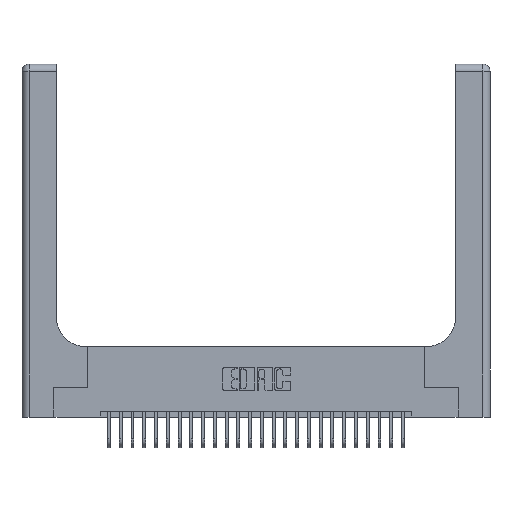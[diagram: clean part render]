
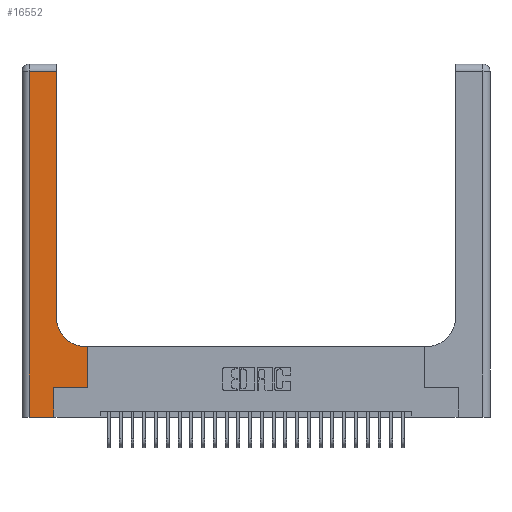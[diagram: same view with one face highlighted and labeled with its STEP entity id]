
A CAD part, top view. The second image highlights one B-rep face of the part: STEP entity #16552.
In plain terms, the highlighted planar face has unit normal (0, 0, 1).
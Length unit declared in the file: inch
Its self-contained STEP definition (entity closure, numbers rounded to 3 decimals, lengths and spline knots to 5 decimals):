
#147 = CARTESIAN_POINT ( 'NONE',  ( 0.269, 0.25, 0.37 ) ) ;
#565 = DIRECTION ( 'NONE',  ( 0., 1., 0. ) ) ;
#669 = ORIENTED_EDGE ( 'NONE', *, *, #23803, .T. ) ;
#1334 = ORIENTED_EDGE ( 'NONE', *, *, #16350, .T. ) ;
#1658 = CARTESIAN_POINT ( 'NONE',  ( 0.2915, 3., 0.37 ) ) ;
#2383 = PLANE ( 'NONE',  #17959 ) ;
#2722 = LINE ( 'NONE', #16464, #17985 ) ;
#2765 = CARTESIAN_POINT ( 'NONE',  ( 0.269, 0., 0.37 ) ) ;
#3053 = EDGE_CURVE ( 'NONE', #5883, #18061, #13501, .T. ) ;
#3487 = CARTESIAN_POINT ( 'NONE',  ( 0.2915, 0.6, 0.37 ) ) ;
#3975 = CARTESIAN_POINT ( 'NONE',  ( 0.2915, 0.85, 0.37 ) ) ;
#4503 = DIRECTION ( 'NONE',  ( -1., 0., 0. ) ) ;
#4833 = LINE ( 'NONE', #11302, #15850 ) ;
#5059 = VERTEX_POINT ( 'NONE', #21029 ) ;
#5406 = FACE_OUTER_BOUND ( 'NONE', #20144, .T. ) ;
#5521 = CARTESIAN_POINT ( 'NONE',  ( 0.5415, 0.6, 0.37 ) ) ;
#5648 = CIRCLE ( 'NONE', #12355, 0.25 ) ;
#5775 = LINE ( 'NONE', #18888, #20976 ) ;
#5845 = VERTEX_POINT ( 'NONE', #2765 ) ;
#5883 = VERTEX_POINT ( 'NONE', #11159 ) ;
#6064 = EDGE_CURVE ( 'NONE', #14129, #5845, #2722, .T. ) ;
#6134 = DIRECTION ( 'NONE',  ( 1., 0., 0. ) ) ;
#7272 = ORIENTED_EDGE ( 'NONE', *, *, #6064, .T. ) ;
#7754 = CARTESIAN_POINT ( 'NONE',  ( 0.5415, 0.85, 0.37 ) ) ;
#7969 = DIRECTION ( 'NONE',  ( 0., 1., 0. ) ) ;
#8744 = VECTOR ( 'NONE', #7969, 39.37008 ) ;
#9002 = EDGE_CURVE ( 'NONE', #21495, #17935, #11755, .T. ) ;
#9151 = CARTESIAN_POINT ( 'NONE',  ( 0.269, 0.25, 0.37 ) ) ;
#9837 = DIRECTION ( 'NONE',  ( 1., 0., 0. ) ) ;
#11151 = ORIENTED_EDGE ( 'NONE', *, *, #9002, .T. ) ;
#11159 = CARTESIAN_POINT ( 'NONE',  ( 0.5585, 0.6, 0.37 ) ) ;
#11218 = DIRECTION ( 'NONE',  ( 1., 0., 0. ) ) ;
#11302 = CARTESIAN_POINT ( 'NONE',  ( 0.06, 3., 0.37 ) ) ;
#11467 = VECTOR ( 'NONE', #565, 39.37008 ) ;
#11755 = LINE ( 'NONE', #9151, #15922 ) ;
#12114 = LINE ( 'NONE', #16015, #11467 ) ;
#12355 = AXIS2_PLACEMENT_3D ( 'NONE', #7754, #22205, #9837 ) ;
#12872 = VECTOR ( 'NONE', #15926, 39.37008 ) ;
#13191 = CARTESIAN_POINT ( 'NONE',  ( 0.06, 0., 0.37 ) ) ;
#13501 = LINE ( 'NONE', #3487, #12872 ) ;
#13969 = CARTESIAN_POINT ( 'NONE',  ( 0.06, 2.94, 0.37 ) ) ;
#14129 = VERTEX_POINT ( 'NONE', #13191 ) ;
#14232 = LINE ( 'NONE', #19849, #8744 ) ;
#14274 = VERTEX_POINT ( 'NONE', #3975 ) ;
#15272 = EDGE_CURVE ( 'NONE', #5845, #21495, #14232, .T. ) ;
#15340 = ORIENTED_EDGE ( 'NONE', *, *, #15272, .T. ) ;
#15850 = VECTOR ( 'NONE', #25762, 39.37008 ) ;
#15922 = VECTOR ( 'NONE', #11218, 39.37008 ) ;
#15926 = DIRECTION ( 'NONE',  ( -1., 0., 0. ) ) ;
#16015 = CARTESIAN_POINT ( 'NONE',  ( 0.5585, 0.25, 0.37 ) ) ;
#16337 = ORIENTED_EDGE ( 'NONE', *, *, #23140, .T. ) ;
#16350 = EDGE_CURVE ( 'NONE', #14274, #5059, #21920, .T. ) ;
#16464 = CARTESIAN_POINT ( 'NONE',  ( 0., 0., 0.37 ) ) ;
#16552 = ADVANCED_FACE ( 'NONE', ( #5406 ), #2383, .F. ) ;
#16932 = DIRECTION ( 'NONE',  ( 0., 0., -1. ) ) ;
#17217 = CARTESIAN_POINT ( 'NONE',  ( 0.5585, 0.25, 0.37 ) ) ;
#17935 = VERTEX_POINT ( 'NONE', #17217 ) ;
#17959 = AXIS2_PLACEMENT_3D ( 'NONE', #22990, #16932, #4503 ) ;
#17985 = VECTOR ( 'NONE', #6134, 39.37008 ) ;
#18061 = VERTEX_POINT ( 'NONE', #5521 ) ;
#18262 = DIRECTION ( 'NONE',  ( 0., 1., 0. ) ) ;
#18888 = CARTESIAN_POINT ( 'NONE',  ( 0., 2.94, 0.37 ) ) ;
#19849 = CARTESIAN_POINT ( 'NONE',  ( 0.269, 0., 0.37 ) ) ;
#20144 = EDGE_LOOP ( 'NONE', ( #1334, #25371, #21809, #7272, #15340, #11151, #669, #26054, #16337 ) ) ;
#20792 = EDGE_CURVE ( 'NONE', #21935, #14129, #4833, .T. ) ;
#20961 = DIRECTION ( 'NONE',  ( -1., 0., 0. ) ) ;
#20976 = VECTOR ( 'NONE', #20961, 39.37008 ) ;
#21029 = CARTESIAN_POINT ( 'NONE',  ( 0.2915, 2.94, 0.37 ) ) ;
#21495 = VERTEX_POINT ( 'NONE', #147 ) ;
#21809 = ORIENTED_EDGE ( 'NONE', *, *, #20792, .T. ) ;
#21920 = LINE ( 'NONE', #1658, #26783 ) ;
#21935 = VERTEX_POINT ( 'NONE', #13969 ) ;
#22205 = DIRECTION ( 'NONE',  ( 0., 0., -1. ) ) ;
#22216 = EDGE_CURVE ( 'NONE', #5059, #21935, #5775, .T. ) ;
#22990 = CARTESIAN_POINT ( 'NONE',  ( 0., 3., 0.37 ) ) ;
#23140 = EDGE_CURVE ( 'NONE', #18061, #14274, #5648, .T. ) ;
#23803 = EDGE_CURVE ( 'NONE', #17935, #5883, #12114, .T. ) ;
#25371 = ORIENTED_EDGE ( 'NONE', *, *, #22216, .T. ) ;
#25762 = DIRECTION ( 'NONE',  ( 0., -1., 0. ) ) ;
#26054 = ORIENTED_EDGE ( 'NONE', *, *, #3053, .T. ) ;
#26783 = VECTOR ( 'NONE', #18262, 39.37008 ) ;
